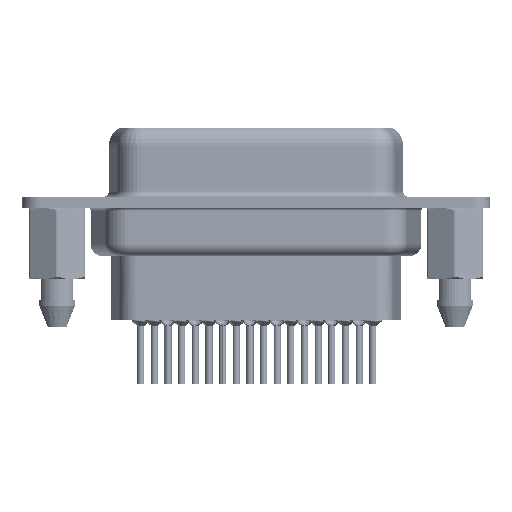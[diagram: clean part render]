
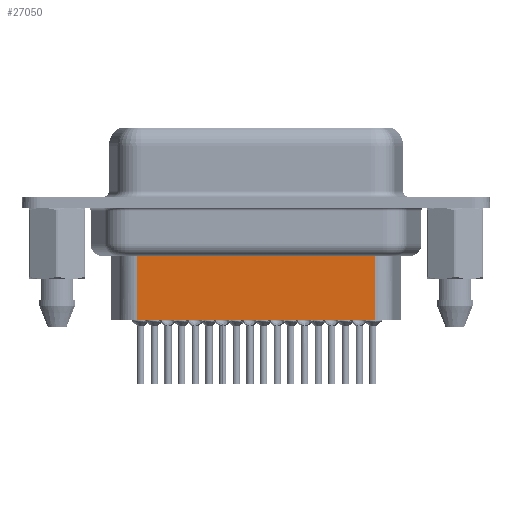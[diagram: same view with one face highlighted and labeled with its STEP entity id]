
A CAD part, front view. The second image highlights one B-rep face of the part: STEP entity #27050.
In plain terms, the highlighted planar face has unit normal (0, -1, 0).
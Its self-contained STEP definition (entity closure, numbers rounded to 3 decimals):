
#122 = VECTOR ( 'NONE', #13612, 1000. ) ;
#616 = CARTESIAN_POINT ( 'NONE',  ( 6.444, -3.5, -4.097 ) ) ;
#1273 = EDGE_LOOP ( 'NONE', ( #25535, #2995, #24192, #9655 ) ) ;
#1882 = VECTOR ( 'NONE', #33018, 1000. ) ;
#2494 = LINE ( 'NONE', #15668, #122 ) ;
#2954 = PLANE ( 'NONE',  #21770 ) ;
#2995 = ORIENTED_EDGE ( 'NONE', *, *, #16083, .T. ) ;
#3670 = EDGE_CURVE ( 'NONE', #20296, #21476, #2494, .T. ) ;
#8155 = LINE ( 'NONE', #616, #32579 ) ;
#8917 = CARTESIAN_POINT ( 'NONE',  ( 6.691, -3.5, -9.85 ) ) ;
#9655 = ORIENTED_EDGE ( 'NONE', *, *, #26760, .F. ) ;
#10698 = FACE_OUTER_BOUND ( 'NONE', #1273, .T. ) ;
#11190 = VERTEX_POINT ( 'NONE', #26692 ) ;
#12500 = EDGE_CURVE ( 'NONE', #19938, #11190, #24795, .T. ) ;
#13612 = DIRECTION ( 'NONE',  ( 0., 0., -1. ) ) ;
#15668 = CARTESIAN_POINT ( 'NONE',  ( 6.691, -3.5, -3.1 ) ) ;
#16083 = EDGE_CURVE ( 'NONE', #19938, #20296, #8155, .T. ) ;
#16313 = VECTOR ( 'NONE', #27115, 1000. ) ;
#16668 = CARTESIAN_POINT ( 'NONE',  ( 26.629, -3.5, -4.097 ) ) ;
#19060 = DIRECTION ( 'NONE',  ( 1., 0., 0. ) ) ;
#19672 = CARTESIAN_POINT ( 'NONE',  ( 26.629, -3.5, -3.1 ) ) ;
#19938 = VERTEX_POINT ( 'NONE', #16668 ) ;
#20296 = VERTEX_POINT ( 'NONE', #28632 ) ;
#21476 = VERTEX_POINT ( 'NONE', #8917 ) ;
#21770 = AXIS2_PLACEMENT_3D ( 'NONE', #24009, #31538, #19060 ) ;
#21985 = CARTESIAN_POINT ( 'NONE',  ( 6.691, -3.5, -9.85 ) ) ;
#23731 = DIRECTION ( 'NONE',  ( -1., 0., 0. ) ) ;
#24009 = CARTESIAN_POINT ( 'NONE',  ( 6.691, -3.5, -3.1 ) ) ;
#24192 = ORIENTED_EDGE ( 'NONE', *, *, #3670, .T. ) ;
#24795 = LINE ( 'NONE', #19672, #1882 ) ;
#25535 = ORIENTED_EDGE ( 'NONE', *, *, #12500, .F. ) ;
#26692 = CARTESIAN_POINT ( 'NONE',  ( 26.629, -3.5, -9.85 ) ) ;
#26760 = EDGE_CURVE ( 'NONE', #11190, #21476, #30206, .T. ) ;
#27050 = ADVANCED_FACE ( 'NONE', ( #10698 ), #2954, .T. ) ;
#27115 = DIRECTION ( 'NONE',  ( -1., 0., 0. ) ) ;
#28632 = CARTESIAN_POINT ( 'NONE',  ( 6.691, -3.5, -4.097 ) ) ;
#30206 = LINE ( 'NONE', #21985, #16313 ) ;
#31538 = DIRECTION ( 'NONE',  ( 0., -1., 0. ) ) ;
#32579 = VECTOR ( 'NONE', #23731, 1000. ) ;
#33018 = DIRECTION ( 'NONE',  ( 0., 0., -1. ) ) ;
